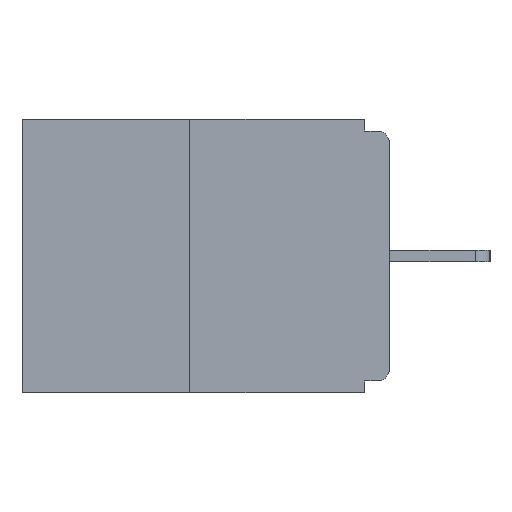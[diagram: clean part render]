
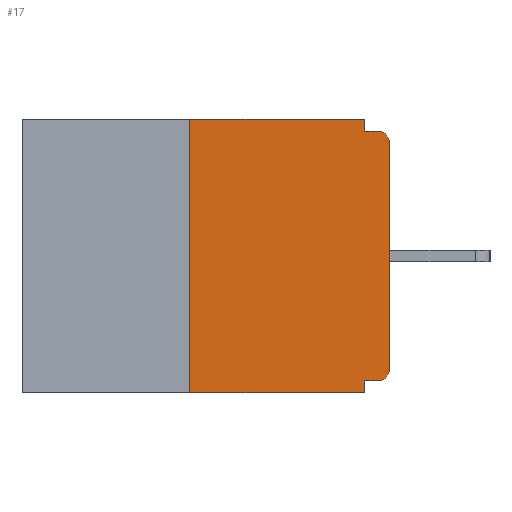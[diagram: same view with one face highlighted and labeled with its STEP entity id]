
A CAD part, left-side view. The second image highlights one B-rep face of the part: STEP entity #17.
In plain terms, the highlighted planar face has unit normal (-1, 0, 0).
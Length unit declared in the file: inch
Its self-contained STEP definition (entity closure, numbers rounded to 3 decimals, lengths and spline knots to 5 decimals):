
#17 = ADVANCED_FACE ( 'NONE', ( #244 ), #11777, .F. ) ;
#21 = VERTEX_POINT ( 'NONE', #4597 ) ;
#244 = FACE_OUTER_BOUND ( 'NONE', #8417, .T. ) ;
#260 = EDGE_CURVE ( 'NONE', #9242, #5850, #1081, .T. ) ;
#376 = LINE ( 'NONE', #6635, #9926 ) ;
#471 = DIRECTION ( 'NONE',  ( 0., 0., 1. ) ) ;
#700 = LINE ( 'NONE', #9756, #10165 ) ;
#752 = ORIENTED_EDGE ( 'NONE', *, *, #260, .T. ) ;
#851 = VERTEX_POINT ( 'NONE', #8229 ) ;
#869 = EDGE_CURVE ( 'NONE', #21, #851, #9669, .T. ) ;
#965 = LINE ( 'NONE', #5789, #10383 ) ;
#1081 = CIRCLE ( 'NONE', #3018, 0.015 ) ;
#1117 = EDGE_CURVE ( 'NONE', #851, #7420, #376, .T. ) ;
#1217 = EDGE_CURVE ( 'NONE', #5850, #7428, #8914, .T. ) ;
#1225 = CARTESIAN_POINT ( 'NONE',  ( 0., 0.015, -0.328 ) ) ;
#1238 = CARTESIAN_POINT ( 'NONE',  ( 0., 0.25, 0. ) ) ;
#1682 = EDGE_CURVE ( 'NONE', #21, #3091, #700, .T. ) ;
#1775 = LINE ( 'NONE', #3958, #4006 ) ;
#1873 = CARTESIAN_POINT ( 'NONE',  ( 0., 0.031, -0.015 ) ) ;
#2275 = LINE ( 'NONE', #5661, #9897 ) ;
#2374 = VERTEX_POINT ( 'NONE', #7978 ) ;
#2479 = CARTESIAN_POINT ( 'NONE',  ( 0., 0.031, -0.343 ) ) ;
#2566 = EDGE_CURVE ( 'NONE', #2374, #3091, #10549, .T. ) ;
#2936 = DIRECTION ( 'NONE',  ( 0., 0., -1. ) ) ;
#3018 = AXIS2_PLACEMENT_3D ( 'NONE', #3930, #6559, #6536 ) ;
#3040 = ORIENTED_EDGE ( 'NONE', *, *, #1682, .T. ) ;
#3091 = VERTEX_POINT ( 'NONE', #2479 ) ;
#3333 = ORIENTED_EDGE ( 'NONE', *, *, #1217, .T. ) ;
#3338 = CARTESIAN_POINT ( 'NONE',  ( 0., 0.015, -0.015 ) ) ;
#3620 = DIRECTION ( 'NONE',  ( 0., 1., 0. ) ) ;
#3739 = CARTESIAN_POINT ( 'NONE',  ( 0., 0., -0.313 ) ) ;
#3780 = VECTOR ( 'NONE', #7969, 39.37008 ) ;
#3930 = CARTESIAN_POINT ( 'NONE',  ( 0., 0.015, -0.313 ) ) ;
#3958 = CARTESIAN_POINT ( 'NONE',  ( 0., 0., -0.328 ) ) ;
#4006 = VECTOR ( 'NONE', #3620, 39.37008 ) ;
#4345 = EDGE_CURVE ( 'NONE', #9242, #2374, #1775, .T. ) ;
#4597 = CARTESIAN_POINT ( 'NONE',  ( 0., 0.25, -0.343 ) ) ;
#4833 = CARTESIAN_POINT ( 'NONE',  ( 0., 0.46, 0. ) ) ;
#4880 = EDGE_CURVE ( 'NONE', #7420, #9854, #965, .T. ) ;
#5295 = ORIENTED_EDGE ( 'NONE', *, *, #1117, .F. ) ;
#5457 = DIRECTION ( 'NONE',  ( 0., -1., 0. ) ) ;
#5463 = EDGE_CURVE ( 'NONE', #7428, #10757, #10502, .T. ) ;
#5661 = CARTESIAN_POINT ( 'NONE',  ( 0., 0., -0.015 ) ) ;
#5789 = CARTESIAN_POINT ( 'NONE',  ( 0., 0.031, 0. ) ) ;
#5850 = VERTEX_POINT ( 'NONE', #3739 ) ;
#5878 = ORIENTED_EDGE ( 'NONE', *, *, #5463, .T. ) ;
#5956 = VECTOR ( 'NONE', #6437, 39.37008 ) ;
#6245 = DIRECTION ( 'NONE',  ( 0., -1., 0. ) ) ;
#6358 = CARTESIAN_POINT ( 'NONE',  ( 0., 0.031, -0.343 ) ) ;
#6437 = DIRECTION ( 'NONE',  ( 0., 0., -1. ) ) ;
#6536 = DIRECTION ( 'NONE',  ( 0., 0., -1. ) ) ;
#6559 = DIRECTION ( 'NONE',  ( -1., 0., 0. ) ) ;
#6635 = CARTESIAN_POINT ( 'NONE',  ( 0., 0.46, 0. ) ) ;
#6669 = DIRECTION ( 'NONE',  ( 0., 0., -1. ) ) ;
#7420 = VERTEX_POINT ( 'NONE', #8935 ) ;
#7428 = VERTEX_POINT ( 'NONE', #8911 ) ;
#7969 = DIRECTION ( 'NONE',  ( 0., 0., 1. ) ) ;
#7978 = CARTESIAN_POINT ( 'NONE',  ( 0., 0.031, -0.328 ) ) ;
#8039 = ORIENTED_EDGE ( 'NONE', *, *, #2566, .F. ) ;
#8047 = CARTESIAN_POINT ( 'NONE',  ( 0., 0., 0. ) ) ;
#8229 = CARTESIAN_POINT ( 'NONE',  ( 0., 0.25, 0. ) ) ;
#8307 = ORIENTED_EDGE ( 'NONE', *, *, #10208, .F. ) ;
#8417 = EDGE_LOOP ( 'NONE', ( #5295, #9947, #3040, #8039, #10198, #752, #3333, #5878, #8307, #10478 ) ) ;
#8464 = AXIS2_PLACEMENT_3D ( 'NONE', #4833, #10218, #2936 ) ;
#8911 = CARTESIAN_POINT ( 'NONE',  ( 0., 0., -0.03 ) ) ;
#8914 = LINE ( 'NONE', #8047, #3780 ) ;
#8935 = CARTESIAN_POINT ( 'NONE',  ( 0., 0.031, 0. ) ) ;
#9242 = VERTEX_POINT ( 'NONE', #1225 ) ;
#9669 = LINE ( 'NONE', #1238, #11642 ) ;
#9700 = CARTESIAN_POINT ( 'NONE',  ( 0., 0.015, -0.03 ) ) ;
#9738 = DIRECTION ( 'NONE',  ( 0., 0., -1. ) ) ;
#9756 = CARTESIAN_POINT ( 'NONE',  ( 0., 0.46, -0.343 ) ) ;
#9763 = DIRECTION ( 'NONE',  ( -1., 0., 0. ) ) ;
#9854 = VERTEX_POINT ( 'NONE', #1873 ) ;
#9897 = VECTOR ( 'NONE', #5457, 39.37008 ) ;
#9926 = VECTOR ( 'NONE', #6245, 39.37008 ) ;
#9947 = ORIENTED_EDGE ( 'NONE', *, *, #869, .F. ) ;
#10165 = VECTOR ( 'NONE', #10778, 39.37008 ) ;
#10198 = ORIENTED_EDGE ( 'NONE', *, *, #4345, .F. ) ;
#10208 = EDGE_CURVE ( 'NONE', #9854, #10757, #2275, .T. ) ;
#10218 = DIRECTION ( 'NONE',  ( 1., 0., 0. ) ) ;
#10383 = VECTOR ( 'NONE', #6669, 39.37008 ) ;
#10478 = ORIENTED_EDGE ( 'NONE', *, *, #4880, .F. ) ;
#10502 = CIRCLE ( 'NONE', #11321, 0.015 ) ;
#10549 = LINE ( 'NONE', #6358, #5956 ) ;
#10757 = VERTEX_POINT ( 'NONE', #3338 ) ;
#10778 = DIRECTION ( 'NONE',  ( 0., -1., 0. ) ) ;
#11321 = AXIS2_PLACEMENT_3D ( 'NONE', #9700, #9763, #9738 ) ;
#11642 = VECTOR ( 'NONE', #471, 39.37008 ) ;
#11777 = PLANE ( 'NONE',  #8464 ) ;
